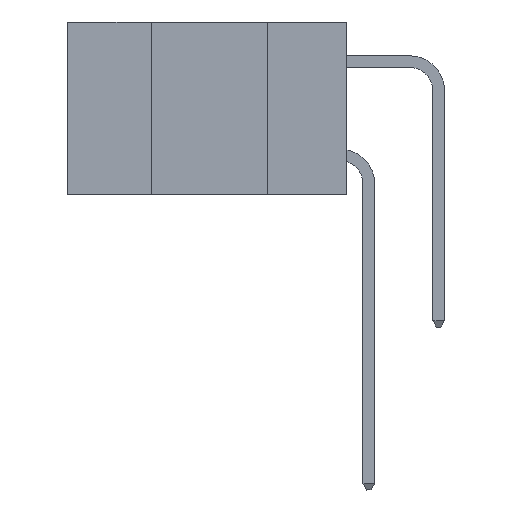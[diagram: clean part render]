
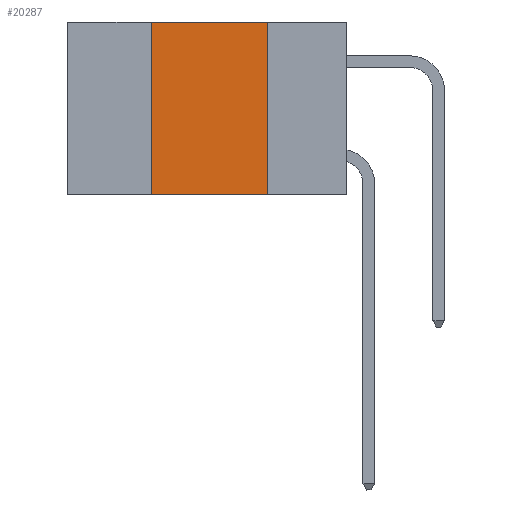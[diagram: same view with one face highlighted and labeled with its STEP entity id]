
A CAD part, left-side view. The second image highlights one B-rep face of the part: STEP entity #20287.
In plain terms, the highlighted planar face has unit normal (-1, 0, 0).
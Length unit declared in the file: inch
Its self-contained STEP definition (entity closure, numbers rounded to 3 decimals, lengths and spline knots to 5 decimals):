
#2569 = AXIS2_PLACEMENT_3D ( 'NONE', #9266, #6129, #37588 ) ;
#3914 = CARTESIAN_POINT ( 'NONE',  ( 0., 0.42, 0. ) ) ;
#3923 = CARTESIAN_POINT ( 'NONE',  ( 0., 0.6, 0. ) ) ;
#6044 = ORIENTED_EDGE ( 'NONE', *, *, #14311, .F. ) ;
#6129 = DIRECTION ( 'NONE',  ( 1., 0., 0. ) ) ;
#6547 = ORIENTED_EDGE ( 'NONE', *, *, #32588, .F. ) ;
#7835 = VERTEX_POINT ( 'NONE', #27381 ) ;
#9266 = CARTESIAN_POINT ( 'NONE',  ( 0., 0.6, 0. ) ) ;
#9618 = CARTESIAN_POINT ( 'NONE',  ( 0., 0.17, 0. ) ) ;
#11547 = VERTEX_POINT ( 'NONE', #20221 ) ;
#11965 = LINE ( 'NONE', #9618, #35316 ) ;
#12446 = FACE_OUTER_BOUND ( 'NONE', #22295, .T. ) ;
#12498 = CARTESIAN_POINT ( 'NONE',  ( 0., 0.6, -0.37 ) ) ;
#13410 = LINE ( 'NONE', #3923, #30525 ) ;
#14311 = EDGE_CURVE ( 'NONE', #17745, #11547, #29243, .T. ) ;
#15754 = DIRECTION ( 'NONE',  ( 0., 0., -1. ) ) ;
#16079 = EDGE_CURVE ( 'NONE', #17745, #7835, #24984, .T. ) ;
#16780 = DIRECTION ( 'NONE',  ( 0., -1., 0. ) ) ;
#17745 = VERTEX_POINT ( 'NONE', #40358 ) ;
#20221 = CARTESIAN_POINT ( 'NONE',  ( 0., 0.42, 0. ) ) ;
#20287 = ADVANCED_FACE ( 'NONE', ( #12446 ), #38190, .F. ) ;
#22295 = EDGE_LOOP ( 'NONE', ( #30039, #6547, #6044, #34416 ) ) ;
#22685 = DIRECTION ( 'NONE',  ( 0., 0., 1. ) ) ;
#24984 = LINE ( 'NONE', #12498, #29288 ) ;
#27381 = CARTESIAN_POINT ( 'NONE',  ( 0., 0.17, -0.37 ) ) ;
#27844 = CARTESIAN_POINT ( 'NONE',  ( 0., 0.17, 0. ) ) ;
#28428 = VECTOR ( 'NONE', #22685, 39.37008 ) ;
#29243 = LINE ( 'NONE', #3914, #28428 ) ;
#29288 = VECTOR ( 'NONE', #31310, 39.37008 ) ;
#30039 = ORIENTED_EDGE ( 'NONE', *, *, #33787, .F. ) ;
#30525 = VECTOR ( 'NONE', #16780, 39.37008 ) ;
#30639 = VERTEX_POINT ( 'NONE', #27844 ) ;
#31310 = DIRECTION ( 'NONE',  ( 0., -1., 0. ) ) ;
#32588 = EDGE_CURVE ( 'NONE', #11547, #30639, #13410, .T. ) ;
#33787 = EDGE_CURVE ( 'NONE', #30639, #7835, #11965, .T. ) ;
#34416 = ORIENTED_EDGE ( 'NONE', *, *, #16079, .T. ) ;
#35316 = VECTOR ( 'NONE', #15754, 39.37008 ) ;
#37588 = DIRECTION ( 'NONE',  ( 0., 0., -1. ) ) ;
#38190 = PLANE ( 'NONE',  #2569 ) ;
#40358 = CARTESIAN_POINT ( 'NONE',  ( 0., 0.42, -0.37 ) ) ;
